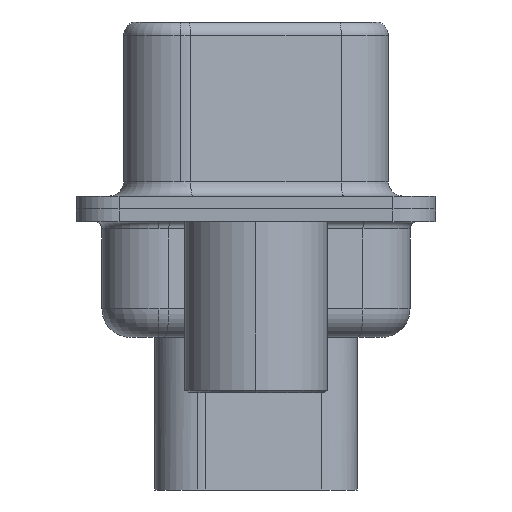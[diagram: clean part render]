
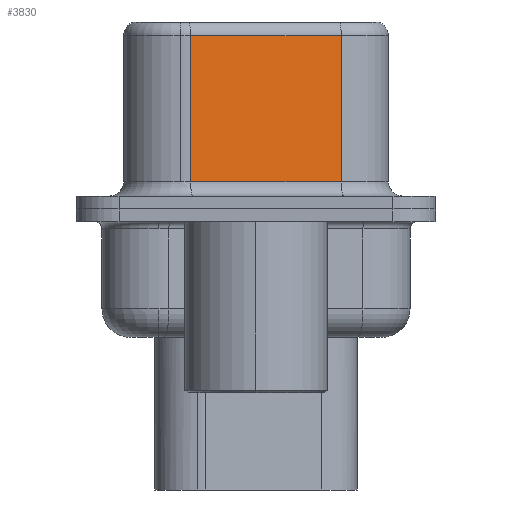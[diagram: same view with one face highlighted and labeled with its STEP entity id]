
A CAD part, left-side view. The second image highlights one B-rep face of the part: STEP entity #3830.
In plain terms, the highlighted planar face has unit normal (-0.985, -0.174, 0).
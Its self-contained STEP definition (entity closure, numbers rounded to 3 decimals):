
#97 = ORIENTED_EDGE ( 'NONE', *, *, #13870, .F. ) ;
#495 = DIRECTION ( 'NONE',  ( 0.174, -0.985, 0. ) ) ;
#3216 = CARTESIAN_POINT ( 'NONE',  ( 4.546, -2.987, 0.95 ) ) ;
#3240 = DIRECTION ( 'NONE',  ( 0., 0., -1. ) ) ;
#3830 = ADVANCED_FACE ( 'NONE', ( #5556 ), #9354, .F. ) ;
#4118 = AXIS2_PLACEMENT_3D ( 'NONE', #14970, #15139, #17603 ) ;
#4241 = CARTESIAN_POINT ( 'NONE',  ( 3.615, 2.293, 6.57 ) ) ;
#4746 = CARTESIAN_POINT ( 'NONE',  ( 3.615, 2.293, 0.95 ) ) ;
#4757 = VERTEX_POINT ( 'NONE', #5395 ) ;
#4797 = VERTEX_POINT ( 'NONE', #11088 ) ;
#4876 = CARTESIAN_POINT ( 'NONE',  ( 4.546, -2.987, 6.07 ) ) ;
#5395 = CARTESIAN_POINT ( 'NONE',  ( 4.546, -2.987, 6.07 ) ) ;
#5408 = VECTOR ( 'NONE', #15639, 1000. ) ;
#5515 = LINE ( 'NONE', #4241, #6638 ) ;
#5556 = FACE_OUTER_BOUND ( 'NONE', #7244, .T. ) ;
#5884 = ORIENTED_EDGE ( 'NONE', *, *, #14275, .T. ) ;
#6029 = VECTOR ( 'NONE', #3240, 1000. ) ;
#6119 = VERTEX_POINT ( 'NONE', #4746 ) ;
#6638 = VECTOR ( 'NONE', #9743, 1000. ) ;
#7244 = EDGE_LOOP ( 'NONE', ( #97, #12693, #9806, #5884 ) ) ;
#8214 = EDGE_CURVE ( 'NONE', #15359, #6119, #5515, .T. ) ;
#9354 = PLANE ( 'NONE',  #4118 ) ;
#9743 = DIRECTION ( 'NONE',  ( 0., 0., -1. ) ) ;
#9806 = ORIENTED_EDGE ( 'NONE', *, *, #8214, .T. ) ;
#10731 = CARTESIAN_POINT ( 'NONE',  ( 3.615, 2.293, 6.07 ) ) ;
#11088 = CARTESIAN_POINT ( 'NONE',  ( 4.546, -2.987, 0.95 ) ) ;
#11244 = VECTOR ( 'NONE', #495, 1000. ) ;
#11438 = LINE ( 'NONE', #3216, #11244 ) ;
#11460 = LINE ( 'NONE', #16979, #6029 ) ;
#11746 = LINE ( 'NONE', #4876, #5408 ) ;
#12693 = ORIENTED_EDGE ( 'NONE', *, *, #17710, .T. ) ;
#13870 = EDGE_CURVE ( 'NONE', #4757, #4797, #11460, .T. ) ;
#14275 = EDGE_CURVE ( 'NONE', #6119, #4797, #11438, .T. ) ;
#14970 = CARTESIAN_POINT ( 'NONE',  ( 4.546, -2.987, 6.57 ) ) ;
#15139 = DIRECTION ( 'NONE',  ( 0.985, 0.174, 0. ) ) ;
#15359 = VERTEX_POINT ( 'NONE', #10731 ) ;
#15639 = DIRECTION ( 'NONE',  ( -0.174, 0.985, 0. ) ) ;
#16979 = CARTESIAN_POINT ( 'NONE',  ( 4.546, -2.987, 6.57 ) ) ;
#17603 = DIRECTION ( 'NONE',  ( -0.174, 0.985, 0. ) ) ;
#17710 = EDGE_CURVE ( 'NONE', #4757, #15359, #11746, .T. ) ;
